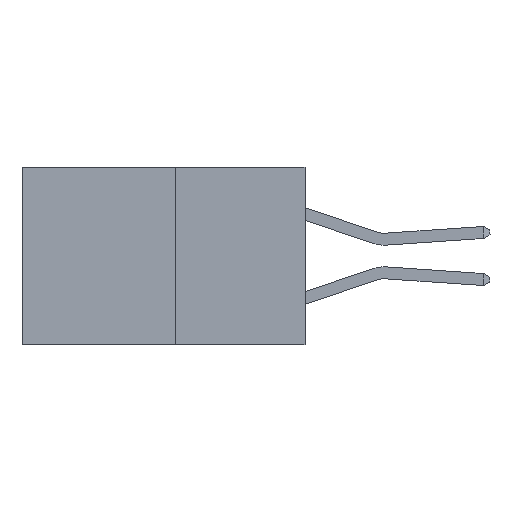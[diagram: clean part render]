
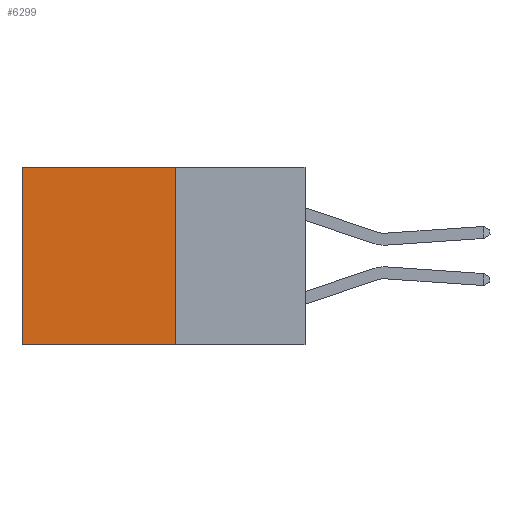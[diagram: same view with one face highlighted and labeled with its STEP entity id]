
A CAD part, left-side view. The second image highlights one B-rep face of the part: STEP entity #6299.
In plain terms, the highlighted planar face has unit normal (-1, 0, 0).
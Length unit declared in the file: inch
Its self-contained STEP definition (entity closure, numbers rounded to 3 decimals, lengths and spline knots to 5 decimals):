
#16 = DIRECTION ( 'NONE',  ( 0., 1., 0. ) ) ;
#286 = DIRECTION ( 'NONE',  ( 0., 1., 0. ) ) ;
#381 = PLANE ( 'NONE',  #795 ) ;
#773 = VERTEX_POINT ( 'NONE', #7546 ) ;
#795 = AXIS2_PLACEMENT_3D ( 'NONE', #5115, #1166, #6689 ) ;
#1166 = DIRECTION ( 'NONE',  ( 1., 0., 0. ) ) ;
#1498 = LINE ( 'NONE', #7894, #5477 ) ;
#1604 = VERTEX_POINT ( 'NONE', #3313 ) ;
#1997 = LINE ( 'NONE', #7822, #4108 ) ;
#2426 = EDGE_CURVE ( 'NONE', #3236, #9096, #4657, .T. ) ;
#2643 = CARTESIAN_POINT ( 'NONE',  ( 0.277, 0.59, -0.37 ) ) ;
#3236 = VERTEX_POINT ( 'NONE', #6476 ) ;
#3313 = CARTESIAN_POINT ( 'NONE',  ( 0.277, 0.27, -0.37 ) ) ;
#3659 = ORIENTED_EDGE ( 'NONE', *, *, #8283, .F. ) ;
#4062 = ORIENTED_EDGE ( 'NONE', *, *, #8220, .T. ) ;
#4108 = VECTOR ( 'NONE', #16, 39.37008 ) ;
#4204 = CARTESIAN_POINT ( 'NONE',  ( 0.277, 0.27, -0.37 ) ) ;
#4382 = EDGE_LOOP ( 'NONE', ( #5230, #5103, #3659, #4062 ) ) ;
#4657 = LINE ( 'NONE', #2643, #6525 ) ;
#4821 = LINE ( 'NONE', #4204, #6676 ) ;
#4966 = FACE_OUTER_BOUND ( 'NONE', #4382, .T. ) ;
#5103 = ORIENTED_EDGE ( 'NONE', *, *, #6496, .F. ) ;
#5115 = CARTESIAN_POINT ( 'NONE',  ( 0.277, 0.27, -0.37 ) ) ;
#5230 = ORIENTED_EDGE ( 'NONE', *, *, #2426, .T. ) ;
#5477 = VECTOR ( 'NONE', #8659, 39.37008 ) ;
#6299 = ADVANCED_FACE ( 'NONE', ( #4966 ), #381, .F. ) ;
#6476 = CARTESIAN_POINT ( 'NONE',  ( 0.277, 0.59, 0. ) ) ;
#6496 = EDGE_CURVE ( 'NONE', #1604, #9096, #4821, .T. ) ;
#6525 = VECTOR ( 'NONE', #6701, 39.37008 ) ;
#6676 = VECTOR ( 'NONE', #286, 39.37008 ) ;
#6689 = DIRECTION ( 'NONE',  ( 0., 0., -1. ) ) ;
#6701 = DIRECTION ( 'NONE',  ( 0., 0., -1. ) ) ;
#7546 = CARTESIAN_POINT ( 'NONE',  ( 0.277, 0.27, 0. ) ) ;
#7822 = CARTESIAN_POINT ( 'NONE',  ( 0.277, 0.27, 0. ) ) ;
#7894 = CARTESIAN_POINT ( 'NONE',  ( 0.277, 0.27, -0.37 ) ) ;
#8220 = EDGE_CURVE ( 'NONE', #773, #3236, #1997, .T. ) ;
#8283 = EDGE_CURVE ( 'NONE', #773, #1604, #1498, .T. ) ;
#8659 = DIRECTION ( 'NONE',  ( 0., 0., -1. ) ) ;
#8846 = CARTESIAN_POINT ( 'NONE',  ( 0.277, 0.59, -0.37 ) ) ;
#9096 = VERTEX_POINT ( 'NONE', #8846 ) ;
